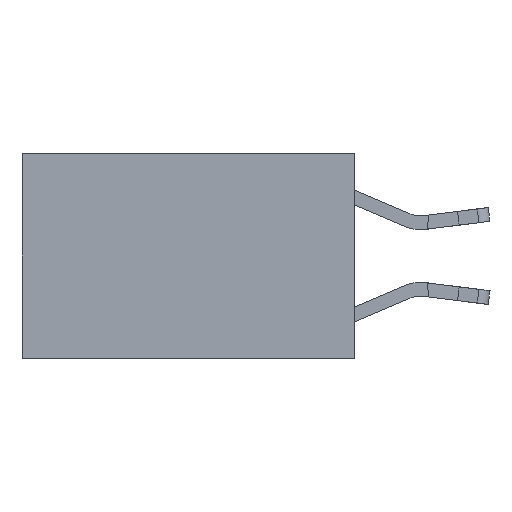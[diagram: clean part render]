
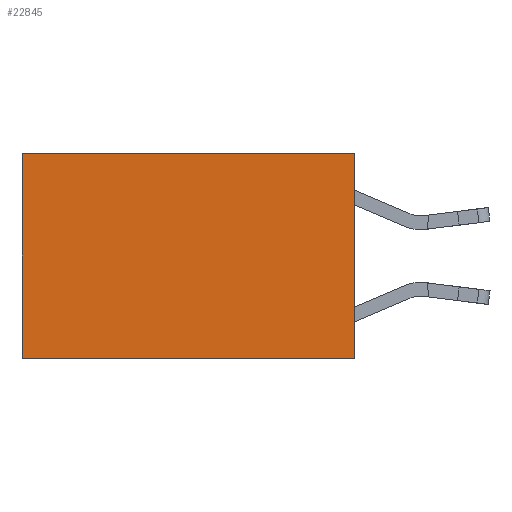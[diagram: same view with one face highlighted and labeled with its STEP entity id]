
A CAD part, left-side view. The second image highlights one B-rep face of the part: STEP entity #22845.
In plain terms, the highlighted planar face has unit normal (-1, 0, 0).
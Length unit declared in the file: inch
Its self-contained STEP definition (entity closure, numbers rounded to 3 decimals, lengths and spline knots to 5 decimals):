
#346 = CARTESIAN_POINT ( 'NONE',  ( 0.2625, 0.6, -0.37 ) ) ;
#483 = AXIS2_PLACEMENT_3D ( 'NONE', #9759, #3349, #18500 ) ;
#779 = VECTOR ( 'NONE', #9550, 39.37008 ) ;
#963 = CARTESIAN_POINT ( 'NONE',  ( 0.2625, 0.6, 0. ) ) ;
#1131 = EDGE_CURVE ( 'NONE', #12698, #26853, #17838, .T. ) ;
#3161 = EDGE_CURVE ( 'NONE', #26853, #11611, #18741, .T. ) ;
#3349 = DIRECTION ( 'NONE',  ( 1., 0., 0. ) ) ;
#4708 = FACE_OUTER_BOUND ( 'NONE', #15577, .T. ) ;
#5158 = LINE ( 'NONE', #963, #779 ) ;
#6359 = CARTESIAN_POINT ( 'NONE',  ( 0.2625, 0., -0.37 ) ) ;
#6415 = ORIENTED_EDGE ( 'NONE', *, *, #3161, .F. ) ;
#8699 = DIRECTION ( 'NONE',  ( 0., 1., 0. ) ) ;
#9550 = DIRECTION ( 'NONE',  ( 0., 0., -1. ) ) ;
#9759 = CARTESIAN_POINT ( 'NONE',  ( 0.2625, 0., 0. ) ) ;
#10240 = VECTOR ( 'NONE', #18200, 39.37008 ) ;
#11611 = VERTEX_POINT ( 'NONE', #346 ) ;
#11978 = DIRECTION ( 'NONE',  ( 0., 0., -1. ) ) ;
#12082 = VECTOR ( 'NONE', #11978, 39.37008 ) ;
#12212 = ORIENTED_EDGE ( 'NONE', *, *, #13664, .T. ) ;
#12698 = VERTEX_POINT ( 'NONE', #21124 ) ;
#13633 = ORIENTED_EDGE ( 'NONE', *, *, #25231, .T. ) ;
#13664 = EDGE_CURVE ( 'NONE', #12698, #15150, #16029, .T. ) ;
#14902 = ORIENTED_EDGE ( 'NONE', *, *, #1131, .F. ) ;
#15150 = VERTEX_POINT ( 'NONE', #20959 ) ;
#15577 = EDGE_LOOP ( 'NONE', ( #13633, #6415, #14902, #12212 ) ) ;
#16029 = LINE ( 'NONE', #26746, #10240 ) ;
#17348 = CARTESIAN_POINT ( 'NONE',  ( 0.2625, 0., 0. ) ) ;
#17838 = LINE ( 'NONE', #17348, #12082 ) ;
#18056 = VECTOR ( 'NONE', #8699, 39.37008 ) ;
#18200 = DIRECTION ( 'NONE',  ( 0., 1., 0. ) ) ;
#18500 = DIRECTION ( 'NONE',  ( 0., 0., -1. ) ) ;
#18741 = LINE ( 'NONE', #6359, #18056 ) ;
#20959 = CARTESIAN_POINT ( 'NONE',  ( 0.2625, 0.6, 0. ) ) ;
#21124 = CARTESIAN_POINT ( 'NONE',  ( 0.2625, 0., 0. ) ) ;
#22709 = PLANE ( 'NONE',  #483 ) ;
#22845 = ADVANCED_FACE ( 'NONE', ( #4708 ), #22709, .F. ) ;
#25231 = EDGE_CURVE ( 'NONE', #15150, #11611, #5158, .T. ) ;
#25849 = CARTESIAN_POINT ( 'NONE',  ( 0.2625, 0., -0.37 ) ) ;
#26746 = CARTESIAN_POINT ( 'NONE',  ( 0.2625, 0., 0. ) ) ;
#26853 = VERTEX_POINT ( 'NONE', #25849 ) ;
